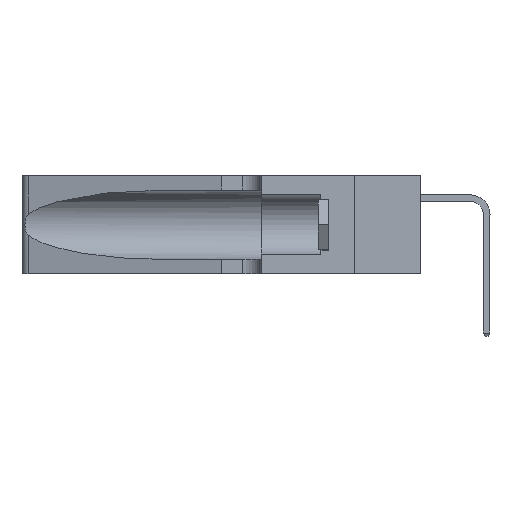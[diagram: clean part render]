
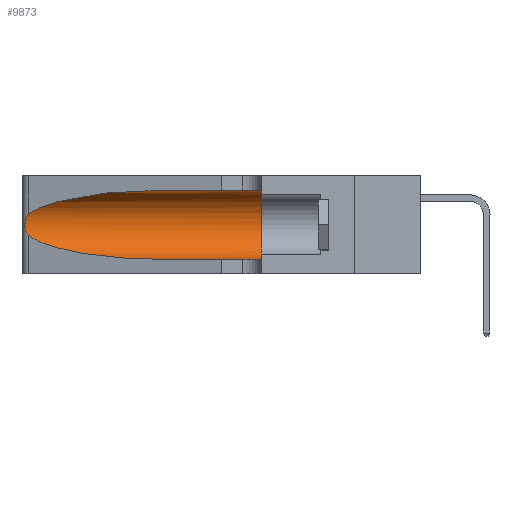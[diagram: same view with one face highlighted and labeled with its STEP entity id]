
A CAD part, left-side view. The second image highlights one B-rep face of the part: STEP entity #9873.
In plain terms, the highlighted cylindrical face has radius 3.308 mm (diameter 6.617 mm), a partial arc.
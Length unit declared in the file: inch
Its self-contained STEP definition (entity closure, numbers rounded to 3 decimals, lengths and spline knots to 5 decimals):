
#140 = CARTESIAN_POINT ( 'NONE',  ( 0.25487, 1.22718, 0.22369 ) ) ;
#462 = ORIENTED_EDGE ( 'NONE', *, *, #18884, .T. ) ;
#1370 = AXIS2_PLACEMENT_3D ( 'NONE', #24544, #6896, #27446 ) ;
#1405 = CARTESIAN_POINT ( 'NONE',  ( 0.1305, 0.72297, 0.05475 ) ) ;
#2548 = LINE ( 'NONE', #31150, #32956 ) ;
#2692 = CARTESIAN_POINT ( 'NONE',  ( 0.1305, 0.72297, 0.31525 ) ) ;
#3279 = CARTESIAN_POINT ( 'NONE',  ( 0.25787, 1.23484, 0.2124 ) ) ;
#3420 = VERTEX_POINT ( 'NONE', #4777 ) ;
#3546 = VERTEX_POINT ( 'NONE', #31790 ) ;
#4777 = CARTESIAN_POINT ( 'NONE',  ( 0.25487, 1.22718, 0.14631 ) ) ;
#6009 = CARTESIAN_POINT ( 'NONE',  ( 0.25555, 1.22994, 0.2215 ) ) ;
#6258 = CARTESIAN_POINT ( 'NONE',  ( 0.26018, 1.23835, 0.19895 ) ) ;
#6395 = CARTESIAN_POINT ( 'NONE',  ( 0.1305, 1.61858, 0.31525 ) ) ;
#6896 = DIRECTION ( 'NONE',  ( 0., 1., 0. ) ) ;
#7424 = EDGE_LOOP ( 'NONE', ( #462, #36616, #32338, #19721, #12142, #7848 ) ) ;
#7848 = ORIENTED_EDGE ( 'NONE', *, *, #32893, .F. ) ;
#8010 = CARTESIAN_POINT ( 'NONE',  ( 0.1305, 0.72297, 0.05475 ) ) ;
#9263 = CARTESIAN_POINT ( 'NONE',  ( 0.26075, 1.23896, 0.178 ) ) ;
#9569 =( BOUNDED_CURVE ( )  B_SPLINE_CURVE ( 3, ( #13214, #30822, #19136, #1405 ),
 .UNSPECIFIED., .F., .T. ) 
 B_SPLINE_CURVE_WITH_KNOTS ( ( 4, 4 ),
 ( 3.44316, 4.71239 ),
 .UNSPECIFIED. ) 
 CURVE ( )  GEOMETRIC_REPRESENTATION_ITEM ( )  RATIONAL_B_SPLINE_CURVE ( ( 1., 0.87, 0.87, 1. ) ) 
 REPRESENTATION_ITEM ( '' )  );
#9873 = ADVANCED_FACE ( 'NONE', ( #14919 ), #29637, .F. ) ;
#11754 =( BOUNDED_CURVE ( )  B_SPLINE_CURVE ( 3, ( #27111, #30099, #12508, #33043 ),
 .UNSPECIFIED., .F., .F. ) 
 B_SPLINE_CURVE_WITH_KNOTS ( ( 4, 4 ),
 ( 1.5708, 2.84003 ),
 .UNSPECIFIED. ) 
 CURVE ( )  GEOMETRIC_REPRESENTATION_ITEM ( )  RATIONAL_B_SPLINE_CURVE ( ( 1., 0.87, 0.87, 1. ) ) 
 REPRESENTATION_ITEM ( '' )  );
#12142 = ORIENTED_EDGE ( 'NONE', *, *, #31202, .F. ) ;
#12211 = CARTESIAN_POINT ( 'NONE',  ( 0.25856, 1.23593, 0.16098 ) ) ;
#12508 = CARTESIAN_POINT ( 'NONE',  ( 0.2373, 1.15595, 0.28018 ) ) ;
#12641 = VERTEX_POINT ( 'NONE', #36269 ) ;
#13214 = CARTESIAN_POINT ( 'NONE',  ( 0.25487, 1.22718, 0.14631 ) ) ;
#14919 = FACE_OUTER_BOUND ( 'NONE', #7424, .T. ) ;
#15037 = EDGE_CURVE ( 'NONE', #24728, #29668, #2548, .T. ) ;
#15113 = CARTESIAN_POINT ( 'NONE',  ( 0.1305, 0.35, 0.05475 ) ) ;
#15152 = CARTESIAN_POINT ( 'NONE',  ( 0.25639, 1.23186, 0.15144 ) ) ;
#17844 = B_SPLINE_CURVE_WITH_KNOTS ( 'NONE', 3,
 ( #140, #6009, #20951, #3279, #23907, #6258, #26838, #9263, #29809, #12211, #32760, #15152, #35707, #18138 ),
 .UNSPECIFIED., .F., .F.,
 ( 4, 2, 2, 2, 2, 2, 4 ),
 ( 0., 0.00027, 0.00053, 0.00107, 0.0016, 0.00187, 0.00214 ),
 .UNSPECIFIED. ) ;
#18138 = CARTESIAN_POINT ( 'NONE',  ( 0.25487, 1.22718, 0.14631 ) ) ;
#18884 = EDGE_CURVE ( 'NONE', #22970, #3546, #11754, .T. ) ;
#19136 = CARTESIAN_POINT ( 'NONE',  ( 0.18966, 0.96281, 0.05475 ) ) ;
#19464 = DIRECTION ( 'NONE',  ( 0., -1., 0. ) ) ;
#19721 = ORIENTED_EDGE ( 'NONE', *, *, #15037, .T. ) ;
#20046 = CARTESIAN_POINT ( 'NONE',  ( 0.1305, 1.61858, 0.185 ) ) ;
#20951 = CARTESIAN_POINT ( 'NONE',  ( 0.25639, 1.23184, 0.21858 ) ) ;
#21074 = DIRECTION ( 'NONE',  ( 0., -1., 0. ) ) ;
#21842 = LINE ( 'NONE', #6395, #28728 ) ;
#22970 = VERTEX_POINT ( 'NONE', #2692 ) ;
#23907 = CARTESIAN_POINT ( 'NONE',  ( 0.25854, 1.2359, 0.20912 ) ) ;
#24544 = CARTESIAN_POINT ( 'NONE',  ( 0.1305, 0.35, 0.185 ) ) ;
#24728 = VERTEX_POINT ( 'NONE', #8010 ) ;
#26838 = CARTESIAN_POINT ( 'NONE',  ( 0.26075, 1.23896, 0.19203 ) ) ;
#27111 = CARTESIAN_POINT ( 'NONE',  ( 0.1305, 0.72297, 0.31525 ) ) ;
#27446 = DIRECTION ( 'NONE',  ( 0., 0., 1. ) ) ;
#28728 = VECTOR ( 'NONE', #21074, 39.37008 ) ;
#28753 = DIRECTION ( 'NONE',  ( 0., 0., -1. ) ) ;
#29637 = CYLINDRICAL_SURFACE ( 'NONE', #31572, 0.13025 ) ;
#29668 = VERTEX_POINT ( 'NONE', #15113 ) ;
#29809 = CARTESIAN_POINT ( 'NONE',  ( 0.26017, 1.23833, 0.17102 ) ) ;
#30099 = CARTESIAN_POINT ( 'NONE',  ( 0.18966, 0.96281, 0.31525 ) ) ;
#30822 = CARTESIAN_POINT ( 'NONE',  ( 0.2373, 1.15595, 0.08982 ) ) ;
#31150 = CARTESIAN_POINT ( 'NONE',  ( 0.1305, 1.61858, 0.05475 ) ) ;
#31202 = EDGE_CURVE ( 'NONE', #12641, #29668, #36696, .T. ) ;
#31306 = EDGE_CURVE ( 'NONE', #3420, #24728, #9569, .T. ) ;
#31572 = AXIS2_PLACEMENT_3D ( 'NONE', #20046, #37612, #28753 ) ;
#31790 = CARTESIAN_POINT ( 'NONE',  ( 0.25487, 1.22718, 0.22369 ) ) ;
#32338 = ORIENTED_EDGE ( 'NONE', *, *, #31306, .T. ) ;
#32760 = CARTESIAN_POINT ( 'NONE',  ( 0.25789, 1.23486, 0.15765 ) ) ;
#32893 = EDGE_CURVE ( 'NONE', #22970, #12641, #21842, .T. ) ;
#32956 = VECTOR ( 'NONE', #19464, 39.37008 ) ;
#33043 = CARTESIAN_POINT ( 'NONE',  ( 0.25487, 1.22718, 0.22369 ) ) ;
#35707 = CARTESIAN_POINT ( 'NONE',  ( 0.25555, 1.22993, 0.14849 ) ) ;
#36269 = CARTESIAN_POINT ( 'NONE',  ( 0.1305, 0.35, 0.31525 ) ) ;
#36616 = ORIENTED_EDGE ( 'NONE', *, *, #37384, .T. ) ;
#36696 = CIRCLE ( 'NONE', #1370, 0.13025 ) ;
#37384 = EDGE_CURVE ( 'NONE', #3546, #3420, #17844, .T. ) ;
#37612 = DIRECTION ( 'NONE',  ( 0., -1., 0. ) ) ;
